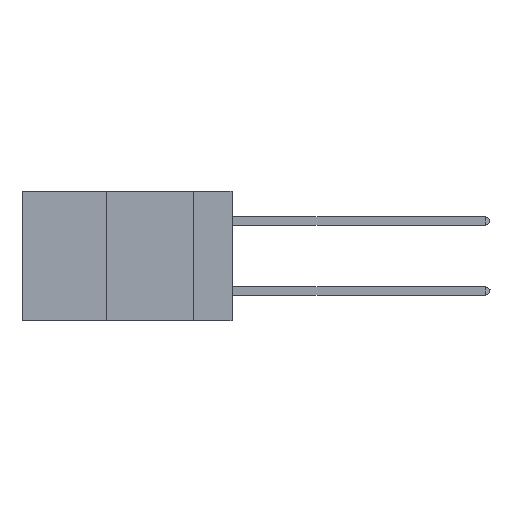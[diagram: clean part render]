
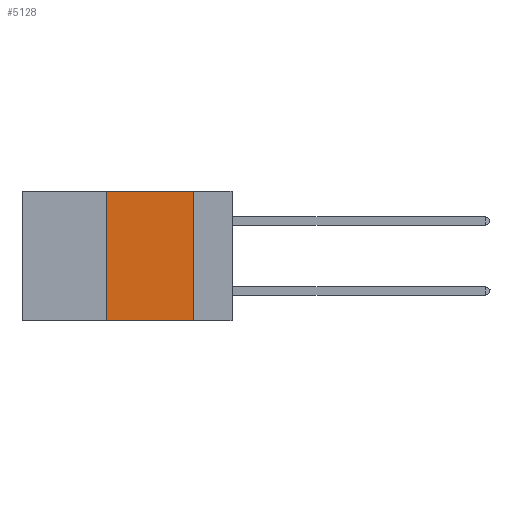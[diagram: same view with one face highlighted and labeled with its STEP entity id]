
A CAD part, left-side view. The second image highlights one B-rep face of the part: STEP entity #5128.
In plain terms, the highlighted planar face has unit normal (-1, 0, 0).
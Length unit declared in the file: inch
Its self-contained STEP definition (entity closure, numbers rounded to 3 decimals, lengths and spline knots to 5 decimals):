
#98 = VERTEX_POINT ( 'NONE', #4764 ) ;
#970 = VERTEX_POINT ( 'NONE', #5961 ) ;
#4335 = DIRECTION ( 'NONE',  ( 0., 0., -1. ) ) ;
#4764 = CARTESIAN_POINT ( 'NONE',  ( 0., 0.36, 0. ) ) ;
#5128 = ADVANCED_FACE ( 'NONE', ( #16356 ), #16059, .F. ) ;
#5326 = VERTEX_POINT ( 'NONE', #11463 ) ;
#5961 = CARTESIAN_POINT ( 'NONE',  ( 0., 0.36, -0.37 ) ) ;
#6045 = DIRECTION ( 'NONE',  ( 0., -1., 0. ) ) ;
#6369 = CARTESIAN_POINT ( 'NONE',  ( 0., 0.6, 0. ) ) ;
#6510 = EDGE_LOOP ( 'NONE', ( #21290, #20286, #9483, #21275 ) ) ;
#7311 = VECTOR ( 'NONE', #4335, 39.37008 ) ;
#7579 = CARTESIAN_POINT ( 'NONE',  ( 0., 0.36, 0. ) ) ;
#7908 = LINE ( 'NONE', #20298, #18875 ) ;
#8235 = CARTESIAN_POINT ( 'NONE',  ( 0., 0.6, -0.37 ) ) ;
#8266 = CARTESIAN_POINT ( 'NONE',  ( 0., 0.11, 0. ) ) ;
#8872 = DIRECTION ( 'NONE',  ( 0., 0., -1. ) ) ;
#9086 = LINE ( 'NONE', #11515, #7311 ) ;
#9483 = ORIENTED_EDGE ( 'NONE', *, *, #12495, .F. ) ;
#11159 = VECTOR ( 'NONE', #13289, 39.37008 ) ;
#11463 = CARTESIAN_POINT ( 'NONE',  ( 0., 0.11, -0.37 ) ) ;
#11515 = CARTESIAN_POINT ( 'NONE',  ( 0., 0.11, 0. ) ) ;
#11985 = EDGE_CURVE ( 'NONE', #21713, #5326, #9086, .T. ) ;
#12495 = EDGE_CURVE ( 'NONE', #970, #98, #21250, .T. ) ;
#13289 = DIRECTION ( 'NONE',  ( 0., 0., 1. ) ) ;
#14354 = DIRECTION ( 'NONE',  ( 1., 0., 0. ) ) ;
#14665 = DIRECTION ( 'NONE',  ( 0., -1., 0. ) ) ;
#15179 = EDGE_CURVE ( 'NONE', #970, #5326, #21114, .T. ) ;
#16059 = PLANE ( 'NONE',  #21877 ) ;
#16356 = FACE_OUTER_BOUND ( 'NONE', #6510, .T. ) ;
#17555 = VECTOR ( 'NONE', #6045, 39.37008 ) ;
#18071 = EDGE_CURVE ( 'NONE', #98, #21713, #7908, .T. ) ;
#18875 = VECTOR ( 'NONE', #14665, 39.37008 ) ;
#20286 = ORIENTED_EDGE ( 'NONE', *, *, #18071, .F. ) ;
#20298 = CARTESIAN_POINT ( 'NONE',  ( 0., 0.6, 0. ) ) ;
#21114 = LINE ( 'NONE', #8235, #17555 ) ;
#21250 = LINE ( 'NONE', #7579, #11159 ) ;
#21275 = ORIENTED_EDGE ( 'NONE', *, *, #15179, .T. ) ;
#21290 = ORIENTED_EDGE ( 'NONE', *, *, #11985, .F. ) ;
#21713 = VERTEX_POINT ( 'NONE', #8266 ) ;
#21877 = AXIS2_PLACEMENT_3D ( 'NONE', #6369, #14354, #8872 ) ;
